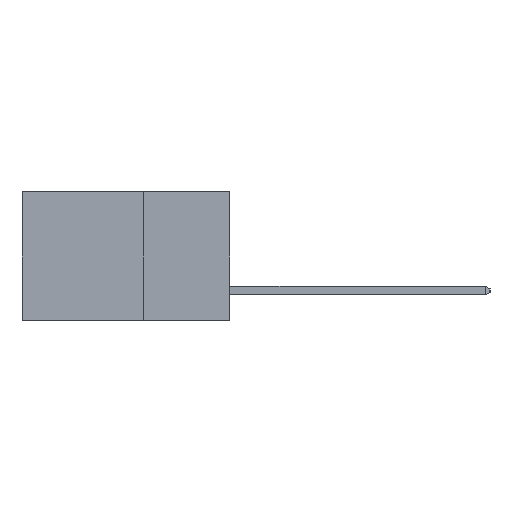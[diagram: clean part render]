
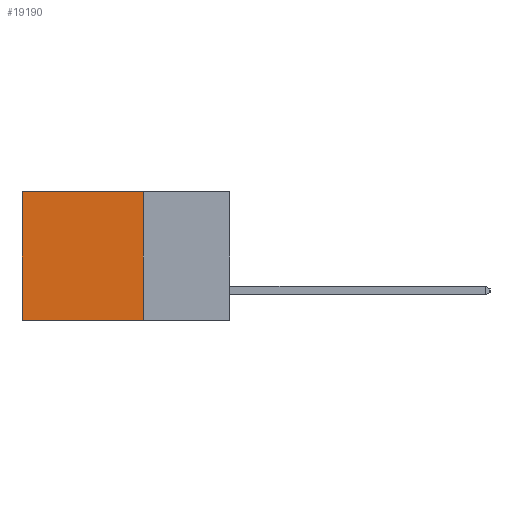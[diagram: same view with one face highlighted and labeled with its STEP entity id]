
A CAD part, left-side view. The second image highlights one B-rep face of the part: STEP entity #19190.
In plain terms, the highlighted planar face has unit normal (-1, 0, 0).
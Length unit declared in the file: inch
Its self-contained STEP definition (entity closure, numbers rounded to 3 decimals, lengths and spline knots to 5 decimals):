
#80 = EDGE_CURVE ( 'NONE', #21341, #2439, #11009, .T. ) ;
#141 = CARTESIAN_POINT ( 'NONE',  ( 0.2615, 0.25, 0. ) ) ;
#1435 = PLANE ( 'NONE',  #21258 ) ;
#2439 = VERTEX_POINT ( 'NONE', #15918 ) ;
#2594 = VECTOR ( 'NONE', #5022, 39.37008 ) ;
#2695 = VECTOR ( 'NONE', #9098, 39.37008 ) ;
#3088 = CARTESIAN_POINT ( 'NONE',  ( 0.2615, 0.6, 0. ) ) ;
#4837 = FACE_OUTER_BOUND ( 'NONE', #6321, .T. ) ;
#4866 = DIRECTION ( 'NONE',  ( 0., 1., 0. ) ) ;
#4993 = CARTESIAN_POINT ( 'NONE',  ( 0.2615, 0.6, -0.37 ) ) ;
#5022 = DIRECTION ( 'NONE',  ( 0., 0., -1. ) ) ;
#5605 = ORIENTED_EDGE ( 'NONE', *, *, #18049, .T. ) ;
#5965 = CARTESIAN_POINT ( 'NONE',  ( 0.2615, 0.25, -0.37 ) ) ;
#6321 = EDGE_LOOP ( 'NONE', ( #19424, #8109, #20071, #5605 ) ) ;
#6408 = VECTOR ( 'NONE', #8931, 39.37008 ) ;
#8109 = ORIENTED_EDGE ( 'NONE', *, *, #19107, .F. ) ;
#8501 = LINE ( 'NONE', #141, #2695 ) ;
#8566 = CARTESIAN_POINT ( 'NONE',  ( 0.2615, 0.25, -0.37 ) ) ;
#8695 = VERTEX_POINT ( 'NONE', #12837 ) ;
#8931 = DIRECTION ( 'NONE',  ( 0., 0., -1. ) ) ;
#9098 = DIRECTION ( 'NONE',  ( 0., 1., 0. ) ) ;
#10071 = CARTESIAN_POINT ( 'NONE',  ( 0.2615, 0.25, 0. ) ) ;
#10316 = DIRECTION ( 'NONE',  ( 1., 0., 0. ) ) ;
#11009 = LINE ( 'NONE', #5965, #6408 ) ;
#11017 = VERTEX_POINT ( 'NONE', #3088 ) ;
#11113 = LINE ( 'NONE', #13465, #15084 ) ;
#11846 = LINE ( 'NONE', #4993, #2594 ) ;
#11917 = EDGE_CURVE ( 'NONE', #11017, #8695, #11846, .T. ) ;
#12837 = CARTESIAN_POINT ( 'NONE',  ( 0.2615, 0.6, -0.37 ) ) ;
#13465 = CARTESIAN_POINT ( 'NONE',  ( 0.2615, 0.25, -0.37 ) ) ;
#15084 = VECTOR ( 'NONE', #4866, 39.37008 ) ;
#15918 = CARTESIAN_POINT ( 'NONE',  ( 0.2615, 0.25, -0.37 ) ) ;
#18049 = EDGE_CURVE ( 'NONE', #21341, #11017, #8501, .T. ) ;
#19107 = EDGE_CURVE ( 'NONE', #2439, #8695, #11113, .T. ) ;
#19190 = ADVANCED_FACE ( 'NONE', ( #4837 ), #1435, .F. ) ;
#19424 = ORIENTED_EDGE ( 'NONE', *, *, #11917, .T. ) ;
#20071 = ORIENTED_EDGE ( 'NONE', *, *, #80, .F. ) ;
#21258 = AXIS2_PLACEMENT_3D ( 'NONE', #8566, #10316, #21917 ) ;
#21341 = VERTEX_POINT ( 'NONE', #10071 ) ;
#21917 = DIRECTION ( 'NONE',  ( 0., 0., -1. ) ) ;
